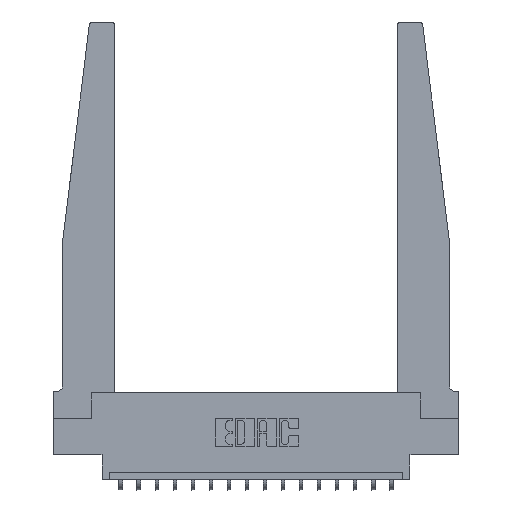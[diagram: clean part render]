
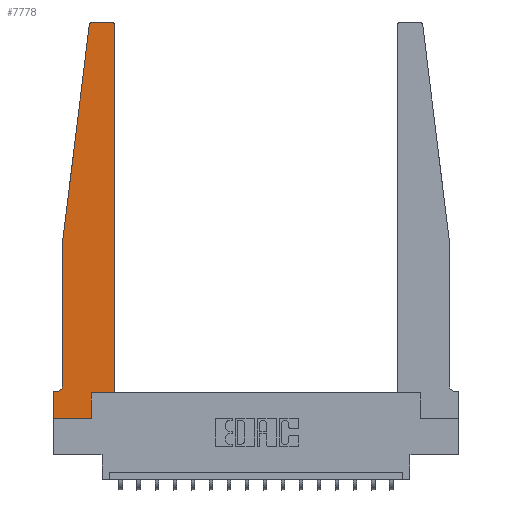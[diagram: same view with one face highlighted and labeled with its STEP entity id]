
A CAD part, top view. The second image highlights one B-rep face of the part: STEP entity #7778.
In plain terms, the highlighted planar face has unit normal (0, 0, 1).
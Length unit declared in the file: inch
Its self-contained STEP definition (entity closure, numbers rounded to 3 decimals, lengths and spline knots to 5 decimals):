
#210 = CARTESIAN_POINT ( 'NONE',  ( 0.27653, 2.75, 0.37 ) ) ;
#477 = VERTEX_POINT ( 'NONE', #4479 ) ;
#994 = VERTEX_POINT ( 'NONE', #17901 ) ;
#1637 = VECTOR ( 'NONE', #6326, 39.37008 ) ;
#2135 = AXIS2_PLACEMENT_3D ( 'NONE', #3799, #15292, #15735 ) ;
#2152 = VERTEX_POINT ( 'NONE', #16626 ) ;
#2155 = EDGE_CURVE ( 'NONE', #9200, #7784, #6152, .T. ) ;
#2347 = VERTEX_POINT ( 'NONE', #5726 ) ;
#2364 = VECTOR ( 'NONE', #16991, 39.37008 ) ;
#2414 = CARTESIAN_POINT ( 'NONE',  ( 0.395, 2.72, 0.37 ) ) ;
#2719 = DIRECTION ( 'NONE',  ( 0., 0., 1. ) ) ;
#2817 = DIRECTION ( 'NONE',  ( 1., 0., 0. ) ) ;
#3001 = CARTESIAN_POINT ( 'NONE',  ( 0.425, 0.18, 0.37 ) ) ;
#3184 = CARTESIAN_POINT ( 'NONE',  ( 0.2605, 0.18, 0.37 ) ) ;
#3367 = DIRECTION ( 'NONE',  ( 0., 1., 0. ) ) ;
#3473 = LINE ( 'NONE', #11218, #2364 ) ;
#3507 = EDGE_CURVE ( 'NONE', #16460, #9200, #10366, .T. ) ;
#3522 = LINE ( 'NONE', #9310, #17598 ) ;
#3570 = VECTOR ( 'NONE', #3367, 39.37008 ) ;
#3659 = AXIS2_PLACEMENT_3D ( 'NONE', #2414, #18313, #8075 ) ;
#3799 = CARTESIAN_POINT ( 'NONE',  ( 0.27653, 2.72, 0.37 ) ) ;
#3815 = LINE ( 'NONE', #9595, #7424 ) ;
#3900 = VECTOR ( 'NONE', #12205, 39.37008 ) ;
#4194 = VECTOR ( 'NONE', #15276, 39.37008 ) ;
#4338 = ORIENTED_EDGE ( 'NONE', *, *, #7748, .T. ) ;
#4458 = LINE ( 'NONE', #15860, #5793 ) ;
#4479 = CARTESIAN_POINT ( 'NONE',  ( 0., 0.1875, 0.37 ) ) ;
#4737 = LINE ( 'NONE', #16353, #16662 ) ;
#5051 = EDGE_CURVE ( 'NONE', #5118, #994, #10295, .T. ) ;
#5118 = VERTEX_POINT ( 'NONE', #210 ) ;
#5726 = CARTESIAN_POINT ( 'NONE',  ( 0.065, 0.2375, 0.37 ) ) ;
#5793 = VECTOR ( 'NONE', #17491, 39.37008 ) ;
#5834 = AXIS2_PLACEMENT_3D ( 'NONE', #16141, #18831, #11716 ) ;
#6011 = EDGE_CURVE ( 'NONE', #6635, #7217, #16730, .T. ) ;
#6152 = LINE ( 'NONE', #13563, #1637 ) ;
#6251 = ORIENTED_EDGE ( 'NONE', *, *, #13313, .T. ) ;
#6326 = DIRECTION ( 'NONE',  ( 1., 0., 0. ) ) ;
#6635 = VERTEX_POINT ( 'NONE', #17601 ) ;
#6649 = CARTESIAN_POINT ( 'NONE',  ( 0.065, 1.25, 0.37 ) ) ;
#6798 = ORIENTED_EDGE ( 'NONE', *, *, #16371, .T. ) ;
#7217 = VERTEX_POINT ( 'NONE', #8975 ) ;
#7424 = VECTOR ( 'NONE', #18382, 39.37008 ) ;
#7511 = EDGE_CURVE ( 'NONE', #2347, #17673, #12816, .T. ) ;
#7748 = EDGE_CURVE ( 'NONE', #7784, #6635, #4737, .T. ) ;
#7778 = ADVANCED_FACE ( 'NONE', ( #15818 ), #13058, .T. ) ;
#7784 = VERTEX_POINT ( 'NONE', #3001 ) ;
#8075 = DIRECTION ( 'NONE',  ( 1., 0., 0. ) ) ;
#8346 = EDGE_CURVE ( 'NONE', #10559, #2347, #3473, .T. ) ;
#8975 = CARTESIAN_POINT ( 'NONE',  ( 0.395, 2.75, 0.37 ) ) ;
#9081 = ORIENTED_EDGE ( 'NONE', *, *, #7511, .T. ) ;
#9136 = EDGE_CURVE ( 'NONE', #7217, #5118, #12389, .T. ) ;
#9164 = EDGE_CURVE ( 'NONE', #2152, #16460, #11073, .T. ) ;
#9200 = VERTEX_POINT ( 'NONE', #13770 ) ;
#9310 = CARTESIAN_POINT ( 'NONE',  ( 0.065, 0.1875, 0.37 ) ) ;
#9595 = CARTESIAN_POINT ( 'NONE',  ( 0.065, 1.25, 0.37 ) ) ;
#9767 = ORIENTED_EDGE ( 'NONE', *, *, #8346, .T. ) ;
#9961 = ORIENTED_EDGE ( 'NONE', *, *, #5051, .T. ) ;
#10295 = CIRCLE ( 'NONE', #2135, 0.03 ) ;
#10366 = LINE ( 'NONE', #3184, #3570 ) ;
#10525 = EDGE_CURVE ( 'NONE', #17673, #477, #3522, .T. ) ;
#10559 = VERTEX_POINT ( 'NONE', #6649 ) ;
#10881 = CARTESIAN_POINT ( 'NONE',  ( 0.015, 0.1875, 0.37 ) ) ;
#11073 = LINE ( 'NONE', #15380, #4194 ) ;
#11218 = CARTESIAN_POINT ( 'NONE',  ( 0.065, 1.25, 0.37 ) ) ;
#11716 = DIRECTION ( 'NONE',  ( -1., 0., 0. ) ) ;
#11777 = ORIENTED_EDGE ( 'NONE', *, *, #2155, .T. ) ;
#12102 = DIRECTION ( 'NONE',  ( 0., 1., 0. ) ) ;
#12205 = DIRECTION ( 'NONE',  ( -1., 0., 0. ) ) ;
#12389 = LINE ( 'NONE', #13961, #3900 ) ;
#12664 = AXIS2_PLACEMENT_3D ( 'NONE', #17177, #2719, #2817 ) ;
#12816 = CIRCLE ( 'NONE', #5834, 0.05 ) ;
#13058 = PLANE ( 'NONE',  #12664 ) ;
#13239 = EDGE_LOOP ( 'NONE', ( #17246, #9961, #6251, #9767, #9081, #13941, #6798, #16322, #15806, #11777, #4338, #18614 ) ) ;
#13313 = EDGE_CURVE ( 'NONE', #994, #10559, #3815, .T. ) ;
#13563 = CARTESIAN_POINT ( 'NONE',  ( 0.425, 0.18, 0.37 ) ) ;
#13770 = CARTESIAN_POINT ( 'NONE',  ( 0.2605, 0.18, 0.37 ) ) ;
#13941 = ORIENTED_EDGE ( 'NONE', *, *, #10525, .T. ) ;
#13961 = CARTESIAN_POINT ( 'NONE',  ( 0.25, 2.75, 0.37 ) ) ;
#15108 = DIRECTION ( 'NONE',  ( -1., 0., 0. ) ) ;
#15276 = DIRECTION ( 'NONE',  ( 1., 0., 0. ) ) ;
#15292 = DIRECTION ( 'NONE',  ( 0., 0., 1. ) ) ;
#15380 = CARTESIAN_POINT ( 'NONE',  ( 0., 0., 0.37 ) ) ;
#15735 = DIRECTION ( 'NONE',  ( 1., 0., 0. ) ) ;
#15806 = ORIENTED_EDGE ( 'NONE', *, *, #3507, .T. ) ;
#15818 = FACE_OUTER_BOUND ( 'NONE', #13239, .T. ) ;
#15860 = CARTESIAN_POINT ( 'NONE',  ( 0., 0., 0.37 ) ) ;
#16141 = CARTESIAN_POINT ( 'NONE',  ( 0.015, 0.2375, 0.37 ) ) ;
#16322 = ORIENTED_EDGE ( 'NONE', *, *, #9164, .T. ) ;
#16343 = CARTESIAN_POINT ( 'NONE',  ( 0.2605, 0., 0.37 ) ) ;
#16353 = CARTESIAN_POINT ( 'NONE',  ( 0.425, 0.18, 0.37 ) ) ;
#16371 = EDGE_CURVE ( 'NONE', #477, #2152, #4458, .T. ) ;
#16460 = VERTEX_POINT ( 'NONE', #16343 ) ;
#16626 = CARTESIAN_POINT ( 'NONE',  ( 0., 0., 0.37 ) ) ;
#16662 = VECTOR ( 'NONE', #12102, 39.37008 ) ;
#16730 = CIRCLE ( 'NONE', #3659, 0.03 ) ;
#16991 = DIRECTION ( 'NONE',  ( 0., -1., 0. ) ) ;
#17177 = CARTESIAN_POINT ( 'NONE',  ( 0., 0.1875, 0.37 ) ) ;
#17246 = ORIENTED_EDGE ( 'NONE', *, *, #9136, .T. ) ;
#17491 = DIRECTION ( 'NONE',  ( 0., -1., 0. ) ) ;
#17598 = VECTOR ( 'NONE', #15108, 39.37008 ) ;
#17601 = CARTESIAN_POINT ( 'NONE',  ( 0.425, 2.72, 0.37 ) ) ;
#17673 = VERTEX_POINT ( 'NONE', #10881 ) ;
#17901 = CARTESIAN_POINT ( 'NONE',  ( 0.24675, 2.72367, 0.37 ) ) ;
#18313 = DIRECTION ( 'NONE',  ( 0., 0., 1. ) ) ;
#18382 = DIRECTION ( 'NONE',  ( -0.122, -0.992, 0. ) ) ;
#18614 = ORIENTED_EDGE ( 'NONE', *, *, #6011, .T. ) ;
#18831 = DIRECTION ( 'NONE',  ( 0., 0., -1. ) ) ;
